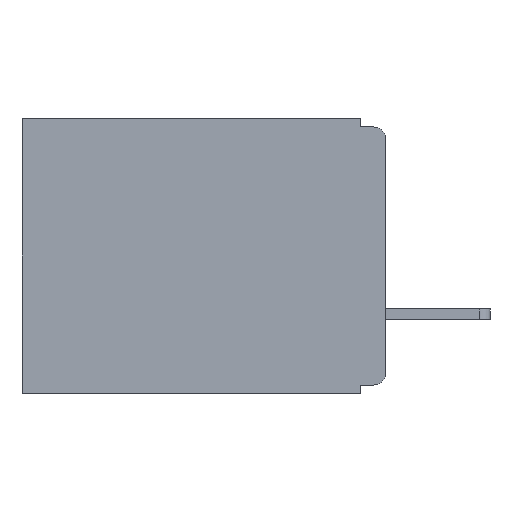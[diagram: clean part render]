
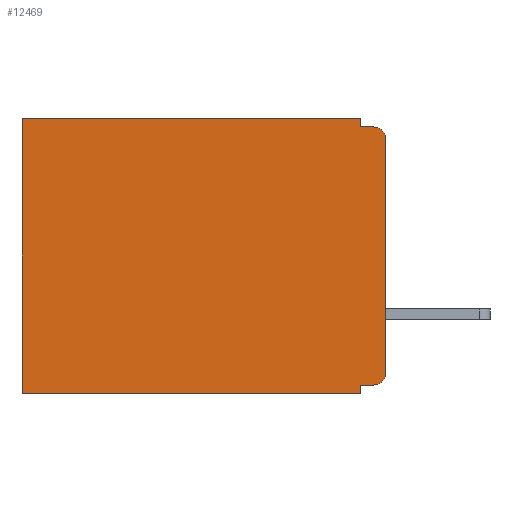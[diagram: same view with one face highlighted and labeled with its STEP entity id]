
A CAD part, left-side view. The second image highlights one B-rep face of the part: STEP entity #12469.
In plain terms, the highlighted planar face has unit normal (-1, 0, 0).
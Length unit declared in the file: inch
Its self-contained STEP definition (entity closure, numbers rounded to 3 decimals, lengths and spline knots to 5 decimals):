
#13 = CARTESIAN_POINT ( 'NONE',  ( 0.3, 0., -0.32 ) ) ;
#822 = DIRECTION ( 'NONE',  ( 0., 1., 0. ) ) ;
#848 = EDGE_CURVE ( 'NONE', #9153, #18034, #19254, .T. ) ;
#1500 = VECTOR ( 'NONE', #23285, 39.37008 ) ;
#2541 = VECTOR ( 'NONE', #10556, 39.37008 ) ;
#2852 = LINE ( 'NONE', #6519, #1500 ) ;
#2972 = CARTESIAN_POINT ( 'NONE',  ( 0.3, 0., -0.33 ) ) ;
#3207 = VECTOR ( 'NONE', #20270, 39.37008 ) ;
#3851 = EDGE_CURVE ( 'NONE', #8495, #13414, #5699, .T. ) ;
#3914 = VERTEX_POINT ( 'NONE', #24744 ) ;
#4277 = AXIS2_PLACEMENT_3D ( 'NONE', #22495, #9911, #24603 ) ;
#4415 = ORIENTED_EDGE ( 'NONE', *, *, #6976, .F. ) ;
#4733 = DIRECTION ( 'NONE',  ( 0., 0., -1. ) ) ;
#5608 = CARTESIAN_POINT ( 'NONE',  ( 0.3, 0.031, 0. ) ) ;
#5699 = CIRCLE ( 'NONE', #8268, 0.015 ) ;
#5770 = ORIENTED_EDGE ( 'NONE', *, *, #22016, .F. ) ;
#5825 = CARTESIAN_POINT ( 'NONE',  ( 0.3, 0., -0.33 ) ) ;
#5828 = CARTESIAN_POINT ( 'NONE',  ( 0.3, 0., -0.33 ) ) ;
#6461 = DIRECTION ( 'NONE',  ( 0., 0., -1. ) ) ;
#6519 = CARTESIAN_POINT ( 'NONE',  ( 0.3, 0., -0.01 ) ) ;
#6649 = ORIENTED_EDGE ( 'NONE', *, *, #23228, .T. ) ;
#6976 = EDGE_CURVE ( 'NONE', #18878, #13414, #15053, .T. ) ;
#7205 = DIRECTION ( 'NONE',  ( 0., 1., 0. ) ) ;
#7394 = CARTESIAN_POINT ( 'NONE',  ( 0.3, 0.031, 0. ) ) ;
#7483 = CARTESIAN_POINT ( 'NONE',  ( 0.3, 0., 0. ) ) ;
#7540 = CARTESIAN_POINT ( 'NONE',  ( 0.3, 0.437, 0. ) ) ;
#7631 = VERTEX_POINT ( 'NONE', #18629 ) ;
#7962 = DIRECTION ( 'NONE',  ( 0., 0., -1. ) ) ;
#8118 = VECTOR ( 'NONE', #7205, 39.37008 ) ;
#8268 = AXIS2_PLACEMENT_3D ( 'NONE', #13554, #23103, #23069 ) ;
#8495 = VERTEX_POINT ( 'NONE', #23628 ) ;
#8927 = CARTESIAN_POINT ( 'NONE',  ( 0.3, 0.031, -0.32 ) ) ;
#9153 = VERTEX_POINT ( 'NONE', #7394 ) ;
#9274 = EDGE_CURVE ( 'NONE', #18878, #3914, #26396, .T. ) ;
#9484 = VECTOR ( 'NONE', #4733, 39.37008 ) ;
#9727 = EDGE_CURVE ( 'NONE', #15220, #26943, #23213, .T. ) ;
#9911 = DIRECTION ( 'NONE',  ( -1., 0., 0. ) ) ;
#10505 = LINE ( 'NONE', #16169, #15422 ) ;
#10556 = DIRECTION ( 'NONE',  ( 0., 1., 0. ) ) ;
#12057 = VECTOR ( 'NONE', #822, 39.37008 ) ;
#12468 = CARTESIAN_POINT ( 'NONE',  ( 0.3, 0., -0.025 ) ) ;
#12469 = ADVANCED_FACE ( 'NONE', ( #18421 ), #26713, .F. ) ;
#13414 = VERTEX_POINT ( 'NONE', #27199 ) ;
#13554 = CARTESIAN_POINT ( 'NONE',  ( 0.3, 0.015, -0.305 ) ) ;
#13977 = VECTOR ( 'NONE', #6461, 39.37008 ) ;
#14074 = DIRECTION ( 'NONE',  ( 0., 0., -1. ) ) ;
#14397 = LINE ( 'NONE', #5608, #3207 ) ;
#14637 = EDGE_CURVE ( 'NONE', #8495, #23878, #19344, .T. ) ;
#15029 = CARTESIAN_POINT ( 'NONE',  ( 0.3, 0.031, -0.33 ) ) ;
#15053 = LINE ( 'NONE', #5825, #9484 ) ;
#15220 = VERTEX_POINT ( 'NONE', #15029 ) ;
#15422 = VECTOR ( 'NONE', #14074, 39.37008 ) ;
#16169 = CARTESIAN_POINT ( 'NONE',  ( 0.3, 0.031, -0.33 ) ) ;
#16645 = EDGE_LOOP ( 'NONE', ( #4415, #21682, #5770, #19160, #26915, #6649, #20112, #25635, #19748, #26210 ) ) ;
#18034 = VERTEX_POINT ( 'NONE', #7540 ) ;
#18113 = CARTESIAN_POINT ( 'NONE',  ( 0.3, 0.437, -0.33 ) ) ;
#18421 = FACE_OUTER_BOUND ( 'NONE', #16645, .T. ) ;
#18629 = CARTESIAN_POINT ( 'NONE',  ( 0.3, 0.031, -0.01 ) ) ;
#18878 = VERTEX_POINT ( 'NONE', #12468 ) ;
#19160 = ORIENTED_EDGE ( 'NONE', *, *, #21698, .F. ) ;
#19254 = LINE ( 'NONE', #7483, #8118 ) ;
#19344 = LINE ( 'NONE', #13, #2541 ) ;
#19748 = ORIENTED_EDGE ( 'NONE', *, *, #14637, .F. ) ;
#20112 = ORIENTED_EDGE ( 'NONE', *, *, #9727, .F. ) ;
#20270 = DIRECTION ( 'NONE',  ( 0., 0., -1. ) ) ;
#20498 = DIRECTION ( 'NONE',  ( 1., 0., 0. ) ) ;
#21094 = CARTESIAN_POINT ( 'NONE',  ( 0.3, 0.437, -0.33 ) ) ;
#21682 = ORIENTED_EDGE ( 'NONE', *, *, #9274, .T. ) ;
#21698 = EDGE_CURVE ( 'NONE', #9153, #7631, #14397, .T. ) ;
#22016 = EDGE_CURVE ( 'NONE', #7631, #3914, #2852, .T. ) ;
#22495 = CARTESIAN_POINT ( 'NONE',  ( 0.3, 0.015, -0.025 ) ) ;
#23069 = DIRECTION ( 'NONE',  ( 0., 0., -1. ) ) ;
#23103 = DIRECTION ( 'NONE',  ( -1., 0., 0. ) ) ;
#23213 = LINE ( 'NONE', #2972, #12057 ) ;
#23228 = EDGE_CURVE ( 'NONE', #18034, #26943, #25146, .T. ) ;
#23285 = DIRECTION ( 'NONE',  ( 0., -1., 0. ) ) ;
#23628 = CARTESIAN_POINT ( 'NONE',  ( 0.3, 0.015, -0.32 ) ) ;
#23878 = VERTEX_POINT ( 'NONE', #8927 ) ;
#24603 = DIRECTION ( 'NONE',  ( 0., 0., -1. ) ) ;
#24744 = CARTESIAN_POINT ( 'NONE',  ( 0.3, 0.015, -0.01 ) ) ;
#25146 = LINE ( 'NONE', #21094, #13977 ) ;
#25635 = ORIENTED_EDGE ( 'NONE', *, *, #26987, .F. ) ;
#26210 = ORIENTED_EDGE ( 'NONE', *, *, #3851, .T. ) ;
#26396 = CIRCLE ( 'NONE', #4277, 0.015 ) ;
#26713 = PLANE ( 'NONE',  #27163 ) ;
#26915 = ORIENTED_EDGE ( 'NONE', *, *, #848, .T. ) ;
#26943 = VERTEX_POINT ( 'NONE', #18113 ) ;
#26987 = EDGE_CURVE ( 'NONE', #23878, #15220, #10505, .T. ) ;
#27163 = AXIS2_PLACEMENT_3D ( 'NONE', #5828, #20498, #7962 ) ;
#27199 = CARTESIAN_POINT ( 'NONE',  ( 0.3, 0., -0.305 ) ) ;
